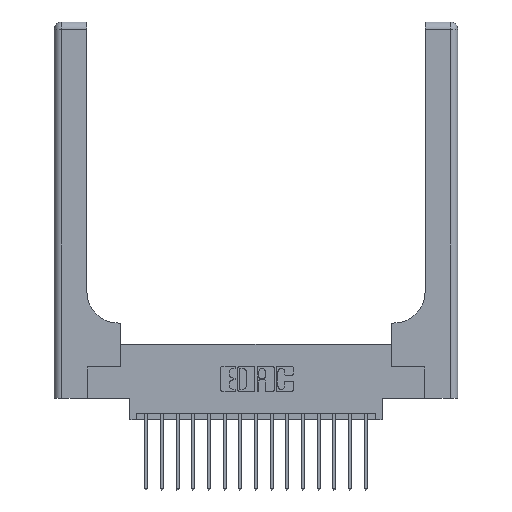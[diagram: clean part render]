
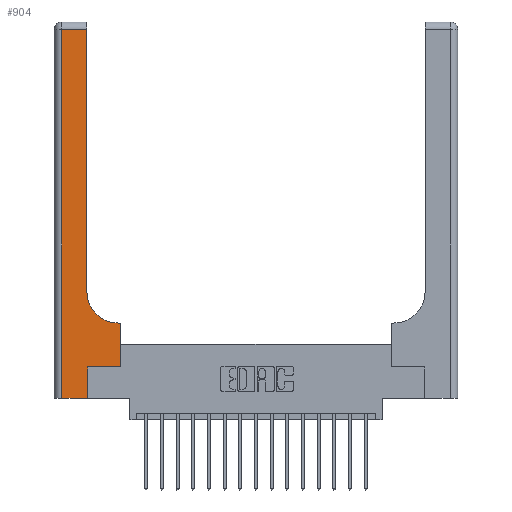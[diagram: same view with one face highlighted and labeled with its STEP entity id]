
A CAD part, top view. The second image highlights one B-rep face of the part: STEP entity #904.
In plain terms, the highlighted planar face has unit normal (0, 0, 1).
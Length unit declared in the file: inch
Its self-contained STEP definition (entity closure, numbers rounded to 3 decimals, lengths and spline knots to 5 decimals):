
#313 = DIRECTION ( 'NONE',  ( 0., 1., 0. ) ) ;
#641 = PLANE ( 'NONE',  #14755 ) ;
#904 = ADVANCED_FACE ( 'NONE', ( #12234 ), #641, .F. ) ;
#1786 = EDGE_CURVE ( 'NONE', #13744, #11167, #9928, .T. ) ;
#2063 = VERTEX_POINT ( 'NONE', #18254 ) ;
#2263 = VECTOR ( 'NONE', #10292, 39.37008 ) ;
#2588 = LINE ( 'NONE', #5881, #2263 ) ;
#2621 = LINE ( 'NONE', #18678, #3992 ) ;
#2693 = CARTESIAN_POINT ( 'NONE',  ( 0.26, 3., 0.37 ) ) ;
#2955 = VERTEX_POINT ( 'NONE', #15364 ) ;
#3033 = VECTOR ( 'NONE', #7417, 39.37008 ) ;
#3679 = VERTEX_POINT ( 'NONE', #13116 ) ;
#3987 = EDGE_CURVE ( 'NONE', #10655, #17220, #8892, .T. ) ;
#3992 = VECTOR ( 'NONE', #8759, 39.37008 ) ;
#4114 = CARTESIAN_POINT ( 'NONE',  ( 0., 2.94, 0.37 ) ) ;
#4222 = DIRECTION ( 'NONE',  ( 1., 0., 0. ) ) ;
#4262 = VECTOR ( 'NONE', #4222, 39.37008 ) ;
#4953 = EDGE_CURVE ( 'NONE', #2955, #13744, #12798, .T. ) ;
#5001 = DIRECTION ( 'NONE',  ( 0., 0., -1. ) ) ;
#5091 = EDGE_CURVE ( 'NONE', #11167, #3679, #2621, .T. ) ;
#5109 = CARTESIAN_POINT ( 'NONE',  ( 0.51, 0.85, 0.37 ) ) ;
#5881 = CARTESIAN_POINT ( 'NONE',  ( 0.06, 3., 0.37 ) ) ;
#5965 = CARTESIAN_POINT ( 'NONE',  ( 0., 0., 0.37 ) ) ;
#6121 = LINE ( 'NONE', #16250, #8498 ) ;
#6429 = ORIENTED_EDGE ( 'NONE', *, *, #11816, .T. ) ;
#6466 = CARTESIAN_POINT ( 'NONE',  ( 0., 3., 0.37 ) ) ;
#6576 = DIRECTION ( 'NONE',  ( 1., 0., 0. ) ) ;
#6610 = EDGE_CURVE ( 'NONE', #2063, #10655, #7258, .T. ) ;
#6721 = ORIENTED_EDGE ( 'NONE', *, *, #6610, .T. ) ;
#7203 = ORIENTED_EDGE ( 'NONE', *, *, #10888, .T. ) ;
#7258 = LINE ( 'NONE', #2693, #13371 ) ;
#7280 = CARTESIAN_POINT ( 'NONE',  ( 0.06, 2.94, 0.37 ) ) ;
#7417 = DIRECTION ( 'NONE',  ( -1., 0., 0. ) ) ;
#7849 = CARTESIAN_POINT ( 'NONE',  ( 0.06, 0., 0.37 ) ) ;
#8228 = DIRECTION ( 'NONE',  ( 0., 0., -1. ) ) ;
#8475 = ORIENTED_EDGE ( 'NONE', *, *, #15264, .T. ) ;
#8498 = VECTOR ( 'NONE', #313, 39.37008 ) ;
#8697 = CARTESIAN_POINT ( 'NONE',  ( 0.265, 0.25, 0.37 ) ) ;
#8759 = DIRECTION ( 'NONE',  ( -1., 0., 0. ) ) ;
#8892 = LINE ( 'NONE', #4114, #3033 ) ;
#9037 = CARTESIAN_POINT ( 'NONE',  ( 0.26, 2.94, 0.37 ) ) ;
#9730 = CARTESIAN_POINT ( 'NONE',  ( 0.528, 0.25, 0.37 ) ) ;
#9928 = LINE ( 'NONE', #9730, #14822 ) ;
#10117 = ORIENTED_EDGE ( 'NONE', *, *, #19189, .T. ) ;
#10292 = DIRECTION ( 'NONE',  ( 0., -1., 0. ) ) ;
#10470 = LINE ( 'NONE', #5965, #4262 ) ;
#10655 = VERTEX_POINT ( 'NONE', #9037 ) ;
#10675 = CARTESIAN_POINT ( 'NONE',  ( 0.528, 0.6, 0.37 ) ) ;
#10804 = AXIS2_PLACEMENT_3D ( 'NONE', #5109, #8228, #6576 ) ;
#10888 = EDGE_CURVE ( 'NONE', #17220, #18933, #2588, .T. ) ;
#11167 = VERTEX_POINT ( 'NONE', #10675 ) ;
#11382 = DIRECTION ( 'NONE',  ( 0., 1., 0. ) ) ;
#11414 = CIRCLE ( 'NONE', #10804, 0.25 ) ;
#11623 = DIRECTION ( 'NONE',  ( 1., 0., 0. ) ) ;
#11816 = EDGE_CURVE ( 'NONE', #17902, #2955, #6121, .T. ) ;
#11900 = ORIENTED_EDGE ( 'NONE', *, *, #3987, .T. ) ;
#12234 = FACE_OUTER_BOUND ( 'NONE', #15849, .T. ) ;
#12798 = LINE ( 'NONE', #8697, #18279 ) ;
#12933 = CARTESIAN_POINT ( 'NONE',  ( 0.528, 0.25, 0.37 ) ) ;
#13116 = CARTESIAN_POINT ( 'NONE',  ( 0.51, 0.6, 0.37 ) ) ;
#13371 = VECTOR ( 'NONE', #17577, 39.37008 ) ;
#13744 = VERTEX_POINT ( 'NONE', #12933 ) ;
#13974 = DIRECTION ( 'NONE',  ( -1., 0., 0. ) ) ;
#14168 = ORIENTED_EDGE ( 'NONE', *, *, #1786, .T. ) ;
#14444 = CARTESIAN_POINT ( 'NONE',  ( 0.265, 0., 0.37 ) ) ;
#14755 = AXIS2_PLACEMENT_3D ( 'NONE', #6466, #5001, #13974 ) ;
#14822 = VECTOR ( 'NONE', #11382, 39.37008 ) ;
#15264 = EDGE_CURVE ( 'NONE', #3679, #2063, #11414, .T. ) ;
#15266 = ORIENTED_EDGE ( 'NONE', *, *, #4953, .T. ) ;
#15364 = CARTESIAN_POINT ( 'NONE',  ( 0.265, 0.25, 0.37 ) ) ;
#15849 = EDGE_LOOP ( 'NONE', ( #6721, #11900, #7203, #10117, #6429, #15266, #14168, #16133, #8475 ) ) ;
#16133 = ORIENTED_EDGE ( 'NONE', *, *, #5091, .T. ) ;
#16250 = CARTESIAN_POINT ( 'NONE',  ( 0.265, 0., 0.37 ) ) ;
#17220 = VERTEX_POINT ( 'NONE', #7280 ) ;
#17577 = DIRECTION ( 'NONE',  ( 0., 1., 0. ) ) ;
#17902 = VERTEX_POINT ( 'NONE', #14444 ) ;
#18254 = CARTESIAN_POINT ( 'NONE',  ( 0.26, 0.85, 0.37 ) ) ;
#18279 = VECTOR ( 'NONE', #11623, 39.37008 ) ;
#18678 = CARTESIAN_POINT ( 'NONE',  ( 0.26, 0.6, 0.37 ) ) ;
#18933 = VERTEX_POINT ( 'NONE', #7849 ) ;
#19189 = EDGE_CURVE ( 'NONE', #18933, #17902, #10470, .T. ) ;
